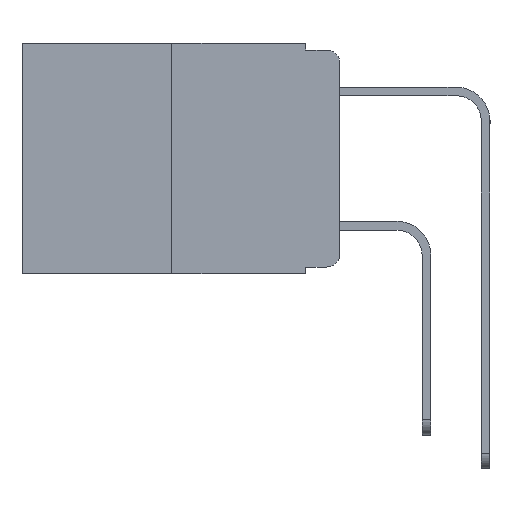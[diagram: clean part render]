
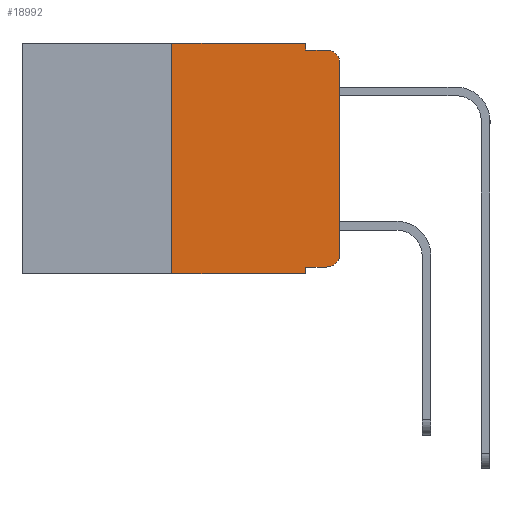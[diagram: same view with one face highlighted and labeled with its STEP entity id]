
A CAD part, left-side view. The second image highlights one B-rep face of the part: STEP entity #18992.
In plain terms, the highlighted planar face has unit normal (-1, 0, 0).
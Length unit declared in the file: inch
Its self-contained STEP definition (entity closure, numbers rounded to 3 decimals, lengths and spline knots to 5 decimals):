
#135 = VECTOR ( 'NONE', #9854, 39.37008 ) ;
#159 = EDGE_CURVE ( 'NONE', #15397, #3772, #17066, .T. ) ;
#163 = DIRECTION ( 'NONE',  ( 0., 0., 1. ) ) ;
#374 = VECTOR ( 'NONE', #163, 39.37008 ) ;
#411 = CARTESIAN_POINT ( 'NONE',  ( 0., 0.051, 0. ) ) ;
#465 = CARTESIAN_POINT ( 'NONE',  ( 0., 0., -0.03 ) ) ;
#617 = ORIENTED_EDGE ( 'NONE', *, *, #1911, .T. ) ;
#693 = VERTEX_POINT ( 'NONE', #10741 ) ;
#806 = DIRECTION ( 'NONE',  ( 0., 0., -1. ) ) ;
#898 = EDGE_CURVE ( 'NONE', #8119, #3772, #12980, .T. ) ;
#1118 = ORIENTED_EDGE ( 'NONE', *, *, #17591, .F. ) ;
#1330 = DIRECTION ( 'NONE',  ( 0., -1., 0. ) ) ;
#1425 = CARTESIAN_POINT ( 'NONE',  ( 0., 0.473, 0. ) ) ;
#1911 = EDGE_CURVE ( 'NONE', #8619, #12965, #18681, .T. ) ;
#2007 = EDGE_CURVE ( 'NONE', #4153, #8119, #9076, .T. ) ;
#2072 = CARTESIAN_POINT ( 'NONE',  ( 0., 0.473, 0. ) ) ;
#3534 = CARTESIAN_POINT ( 'NONE',  ( 0., 0.051, -0.343 ) ) ;
#3575 = DIRECTION ( 'NONE',  ( 0., 0., 1. ) ) ;
#3665 = DIRECTION ( 'NONE',  ( -1., 0., 0. ) ) ;
#3772 = VERTEX_POINT ( 'NONE', #20203 ) ;
#3822 = AXIS2_PLACEMENT_3D ( 'NONE', #2072, #16323, #7030 ) ;
#4052 = ORIENTED_EDGE ( 'NONE', *, *, #898, .T. ) ;
#4096 = DIRECTION ( 'NONE',  ( 0., -1., 0. ) ) ;
#4127 = ORIENTED_EDGE ( 'NONE', *, *, #19611, .F. ) ;
#4153 = VERTEX_POINT ( 'NONE', #19554 ) ;
#4187 = ORIENTED_EDGE ( 'NONE', *, *, #6281, .F. ) ;
#4231 = CARTESIAN_POINT ( 'NONE',  ( 0., 0.02, -0.333 ) ) ;
#4295 = ORIENTED_EDGE ( 'NONE', *, *, #159, .F. ) ;
#4586 = ORIENTED_EDGE ( 'NONE', *, *, #16578, .F. ) ;
#5398 = AXIS2_PLACEMENT_3D ( 'NONE', #14372, #7082, #13731 ) ;
#5405 = PLANE ( 'NONE',  #3822 ) ;
#5644 = VECTOR ( 'NONE', #14148, 39.37008 ) ;
#5900 = LINE ( 'NONE', #8079, #17795 ) ;
#6077 = EDGE_LOOP ( 'NONE', ( #18420, #4052, #4295, #4127, #4187, #1118, #617, #4586, #8313, #6418 ) ) ;
#6281 = EDGE_CURVE ( 'NONE', #693, #19787, #10370, .T. ) ;
#6346 = VECTOR ( 'NONE', #4096, 39.37008 ) ;
#6418 = ORIENTED_EDGE ( 'NONE', *, *, #13479, .T. ) ;
#7030 = DIRECTION ( 'NONE',  ( 0., 0., -1. ) ) ;
#7082 = DIRECTION ( 'NONE',  ( -1., 0., 0. ) ) ;
#7285 = VECTOR ( 'NONE', #806, 39.37008 ) ;
#7315 = VECTOR ( 'NONE', #1330, 39.37008 ) ;
#7347 = CARTESIAN_POINT ( 'NONE',  ( 0., 0.051, -0.333 ) ) ;
#8079 = CARTESIAN_POINT ( 'NONE',  ( 0., 0.051, 0. ) ) ;
#8119 = VERTEX_POINT ( 'NONE', #465 ) ;
#8175 = CARTESIAN_POINT ( 'NONE',  ( 0., 0.25, -0.343 ) ) ;
#8313 = ORIENTED_EDGE ( 'NONE', *, *, #14506, .T. ) ;
#8619 = VERTEX_POINT ( 'NONE', #8175 ) ;
#8984 = LINE ( 'NONE', #11548, #12608 ) ;
#9076 = LINE ( 'NONE', #11546, #374 ) ;
#9678 = DIRECTION ( 'NONE',  ( 0., 0., -1. ) ) ;
#9706 = CARTESIAN_POINT ( 'NONE',  ( 0., 0.473, -0.343 ) ) ;
#9854 = DIRECTION ( 'NONE',  ( 0., -1., 0. ) ) ;
#10370 = LINE ( 'NONE', #1425, #5644 ) ;
#10741 = CARTESIAN_POINT ( 'NONE',  ( 0., 0.25, 0. ) ) ;
#11354 = VERTEX_POINT ( 'NONE', #4231 ) ;
#11546 = CARTESIAN_POINT ( 'NONE',  ( 0., 0., 0. ) ) ;
#11548 = CARTESIAN_POINT ( 'NONE',  ( 0., 0.25, 0. ) ) ;
#11772 = CIRCLE ( 'NONE', #16917, 0.02 ) ;
#12528 = VERTEX_POINT ( 'NONE', #7347 ) ;
#12608 = VECTOR ( 'NONE', #3575, 39.37008 ) ;
#12965 = VERTEX_POINT ( 'NONE', #3534 ) ;
#12980 = CIRCLE ( 'NONE', #5398, 0.02 ) ;
#13163 = CARTESIAN_POINT ( 'NONE',  ( 0., 0.02, -0.313 ) ) ;
#13479 = EDGE_CURVE ( 'NONE', #11354, #4153, #11772, .T. ) ;
#13494 = CARTESIAN_POINT ( 'NONE',  ( 0., 0.051, -0.01 ) ) ;
#13731 = DIRECTION ( 'NONE',  ( 0., 0., -1. ) ) ;
#14148 = DIRECTION ( 'NONE',  ( 0., -1., 0. ) ) ;
#14372 = CARTESIAN_POINT ( 'NONE',  ( 0., 0.02, -0.03 ) ) ;
#14506 = EDGE_CURVE ( 'NONE', #12528, #11354, #20060, .T. ) ;
#14708 = DIRECTION ( 'NONE',  ( 0., 0., -1. ) ) ;
#15397 = VERTEX_POINT ( 'NONE', #17171 ) ;
#15526 = LINE ( 'NONE', #19661, #7285 ) ;
#16323 = DIRECTION ( 'NONE',  ( 1., 0., 0. ) ) ;
#16578 = EDGE_CURVE ( 'NONE', #12528, #12965, #15526, .T. ) ;
#16917 = AXIS2_PLACEMENT_3D ( 'NONE', #13163, #3665, #14708 ) ;
#17066 = LINE ( 'NONE', #13494, #135 ) ;
#17171 = CARTESIAN_POINT ( 'NONE',  ( 0., 0.051, -0.01 ) ) ;
#17591 = EDGE_CURVE ( 'NONE', #8619, #693, #8984, .T. ) ;
#17795 = VECTOR ( 'NONE', #9678, 39.37008 ) ;
#18070 = FACE_OUTER_BOUND ( 'NONE', #6077, .T. ) ;
#18420 = ORIENTED_EDGE ( 'NONE', *, *, #2007, .T. ) ;
#18681 = LINE ( 'NONE', #9706, #6346 ) ;
#18992 = ADVANCED_FACE ( 'NONE', ( #18070 ), #5405, .F. ) ;
#19554 = CARTESIAN_POINT ( 'NONE',  ( 0., 0., -0.313 ) ) ;
#19611 = EDGE_CURVE ( 'NONE', #19787, #15397, #5900, .T. ) ;
#19661 = CARTESIAN_POINT ( 'NONE',  ( 0., 0.051, 0. ) ) ;
#19787 = VERTEX_POINT ( 'NONE', #411 ) ;
#20060 = LINE ( 'NONE', #20104, #7315 ) ;
#20104 = CARTESIAN_POINT ( 'NONE',  ( 0., 0.051, -0.333 ) ) ;
#20203 = CARTESIAN_POINT ( 'NONE',  ( 0., 0.02, -0.01 ) ) ;
